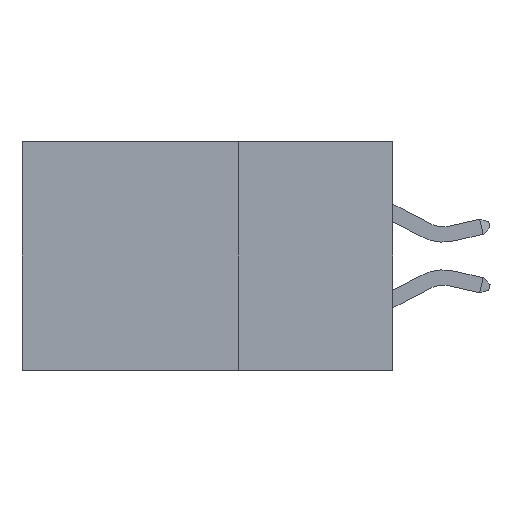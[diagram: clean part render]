
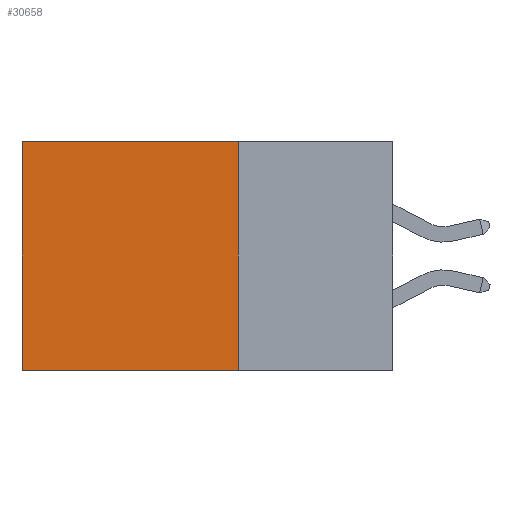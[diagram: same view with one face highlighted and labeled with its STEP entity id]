
A CAD part, left-side view. The second image highlights one B-rep face of the part: STEP entity #30658.
In plain terms, the highlighted planar face has unit normal (-1, 0, 0).
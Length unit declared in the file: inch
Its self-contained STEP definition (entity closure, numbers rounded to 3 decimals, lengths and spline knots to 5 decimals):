
#592 = VECTOR ( 'NONE', #23574, 39.37008 ) ;
#1081 = LINE ( 'NONE', #16478, #26191 ) ;
#3289 = CARTESIAN_POINT ( 'NONE',  ( 0.2875, 0.25, 0. ) ) ;
#3448 = ORIENTED_EDGE ( 'NONE', *, *, #31707, .T. ) ;
#5362 = VECTOR ( 'NONE', #19981, 39.37008 ) ;
#7535 = PLANE ( 'NONE',  #17715 ) ;
#11351 = CARTESIAN_POINT ( 'NONE',  ( 0.2875, 0.6, -0.37 ) ) ;
#11891 = LINE ( 'NONE', #34277, #25506 ) ;
#13391 = DIRECTION ( 'NONE',  ( 0., 0., -1. ) ) ;
#15434 = ORIENTED_EDGE ( 'NONE', *, *, #25462, .F. ) ;
#15762 = FACE_OUTER_BOUND ( 'NONE', #31648, .T. ) ;
#16478 = CARTESIAN_POINT ( 'NONE',  ( 0.2875, 0.6, 0. ) ) ;
#17188 = CARTESIAN_POINT ( 'NONE',  ( 0.2875, 0.25, 0. ) ) ;
#17224 = ORIENTED_EDGE ( 'NONE', *, *, #34516, .F. ) ;
#17715 = AXIS2_PLACEMENT_3D ( 'NONE', #27850, #30775, #13391 ) ;
#19298 = EDGE_CURVE ( 'NONE', #34741, #31497, #27644, .T. ) ;
#19398 = DIRECTION ( 'NONE',  ( 0., 0., -1. ) ) ;
#19981 = DIRECTION ( 'NONE',  ( 0., 1., 0. ) ) ;
#20646 = CARTESIAN_POINT ( 'NONE',  ( 0.2875, 0.25, 0. ) ) ;
#23574 = DIRECTION ( 'NONE',  ( 0., 0., -1. ) ) ;
#23872 = LINE ( 'NONE', #20646, #592 ) ;
#25462 = EDGE_CURVE ( 'NONE', #34741, #29701, #23872, .T. ) ;
#25504 = ORIENTED_EDGE ( 'NONE', *, *, #19298, .T. ) ;
#25506 = VECTOR ( 'NONE', #37172, 39.37008 ) ;
#26191 = VECTOR ( 'NONE', #19398, 39.37008 ) ;
#26658 = CARTESIAN_POINT ( 'NONE',  ( 0.2875, 0.25, -0.37 ) ) ;
#27138 = CARTESIAN_POINT ( 'NONE',  ( 0.2875, 0.6, 0. ) ) ;
#27644 = LINE ( 'NONE', #17188, #5362 ) ;
#27850 = CARTESIAN_POINT ( 'NONE',  ( 0.2875, 0.25, 0. ) ) ;
#29701 = VERTEX_POINT ( 'NONE', #26658 ) ;
#30658 = ADVANCED_FACE ( 'NONE', ( #15762 ), #7535, .F. ) ;
#30775 = DIRECTION ( 'NONE',  ( 1., 0., 0. ) ) ;
#30870 = VERTEX_POINT ( 'NONE', #11351 ) ;
#31497 = VERTEX_POINT ( 'NONE', #27138 ) ;
#31648 = EDGE_LOOP ( 'NONE', ( #3448, #17224, #15434, #25504 ) ) ;
#31707 = EDGE_CURVE ( 'NONE', #31497, #30870, #1081, .T. ) ;
#34277 = CARTESIAN_POINT ( 'NONE',  ( 0.2875, 0.25, -0.37 ) ) ;
#34516 = EDGE_CURVE ( 'NONE', #29701, #30870, #11891, .T. ) ;
#34741 = VERTEX_POINT ( 'NONE', #3289 ) ;
#37172 = DIRECTION ( 'NONE',  ( 0., 1., 0. ) ) ;
